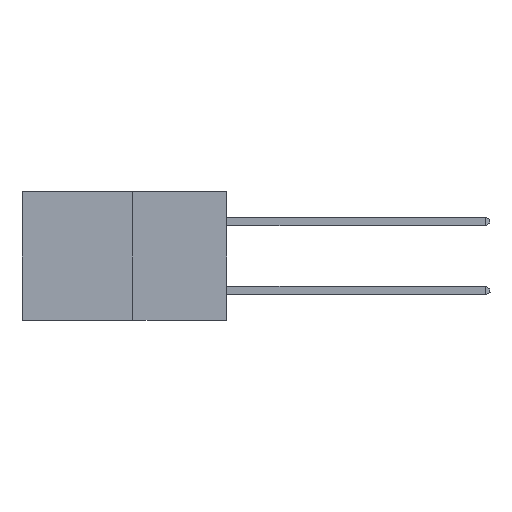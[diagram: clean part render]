
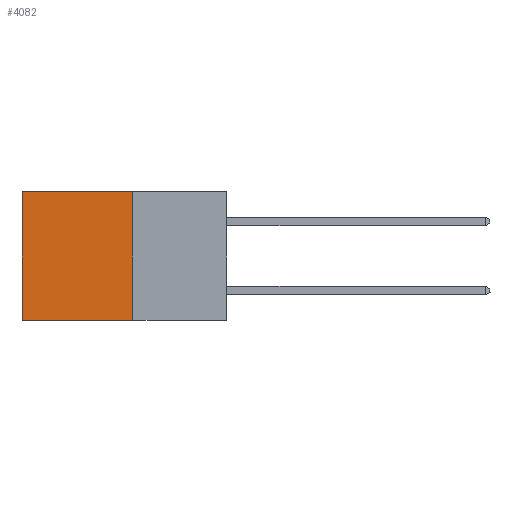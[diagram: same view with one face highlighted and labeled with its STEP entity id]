
A CAD part, left-side view. The second image highlights one B-rep face of the part: STEP entity #4082.
In plain terms, the highlighted planar face has unit normal (-1, 0, 0).
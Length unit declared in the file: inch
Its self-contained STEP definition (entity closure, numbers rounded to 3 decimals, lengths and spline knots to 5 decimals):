
#1865 = LINE ( 'NONE', #2295, #23714 ) ;
#2295 = CARTESIAN_POINT ( 'NONE',  ( 0.277, 0.27, -0.37 ) ) ;
#4072 = CARTESIAN_POINT ( 'NONE',  ( 0.277, 0.59, -0.37 ) ) ;
#4082 = ADVANCED_FACE ( 'NONE', ( #4358 ), #12437, .F. ) ;
#4358 = FACE_OUTER_BOUND ( 'NONE', #25690, .T. ) ;
#4457 = EDGE_CURVE ( 'NONE', #16605, #13602, #10666, .T. ) ;
#4760 = ORIENTED_EDGE ( 'NONE', *, *, #11035, .F. ) ;
#4794 = CARTESIAN_POINT ( 'NONE',  ( 0.277, 0.59, 0. ) ) ;
#5873 = DIRECTION ( 'NONE',  ( 0., 1., 0. ) ) ;
#6000 = CARTESIAN_POINT ( 'NONE',  ( 0.277, 0.27, 0. ) ) ;
#8192 = LINE ( 'NONE', #19286, #25667 ) ;
#9431 = DIRECTION ( 'NONE',  ( 0., 1., 0. ) ) ;
#10104 = AXIS2_PLACEMENT_3D ( 'NONE', #12379, #12317, #12293 ) ;
#10666 = LINE ( 'NONE', #6000, #15632 ) ;
#10964 = LINE ( 'NONE', #24340, #11753 ) ;
#11035 = EDGE_CURVE ( 'NONE', #25923, #20314, #10964, .T. ) ;
#11753 = VECTOR ( 'NONE', #9431, 39.37008 ) ;
#12293 = DIRECTION ( 'NONE',  ( 0., 0., -1. ) ) ;
#12317 = DIRECTION ( 'NONE',  ( 1., 0., 0. ) ) ;
#12379 = CARTESIAN_POINT ( 'NONE',  ( 0.277, 0.27, -0.37 ) ) ;
#12437 = PLANE ( 'NONE',  #10104 ) ;
#13024 = DIRECTION ( 'NONE',  ( 0., 0., -1. ) ) ;
#13602 = VERTEX_POINT ( 'NONE', #4794 ) ;
#15466 = EDGE_CURVE ( 'NONE', #16605, #25923, #1865, .T. ) ;
#15632 = VECTOR ( 'NONE', #5873, 39.37008 ) ;
#15889 = EDGE_CURVE ( 'NONE', #13602, #20314, #8192, .T. ) ;
#16514 = ORIENTED_EDGE ( 'NONE', *, *, #15466, .F. ) ;
#16605 = VERTEX_POINT ( 'NONE', #17299 ) ;
#17299 = CARTESIAN_POINT ( 'NONE',  ( 0.277, 0.27, 0. ) ) ;
#19286 = CARTESIAN_POINT ( 'NONE',  ( 0.277, 0.59, -0.37 ) ) ;
#20314 = VERTEX_POINT ( 'NONE', #4072 ) ;
#20884 = ORIENTED_EDGE ( 'NONE', *, *, #4457, .T. ) ;
#22381 = ORIENTED_EDGE ( 'NONE', *, *, #15889, .T. ) ;
#23476 = DIRECTION ( 'NONE',  ( 0., 0., -1. ) ) ;
#23714 = VECTOR ( 'NONE', #23476, 39.37008 ) ;
#24340 = CARTESIAN_POINT ( 'NONE',  ( 0.277, 0.27, -0.37 ) ) ;
#24460 = CARTESIAN_POINT ( 'NONE',  ( 0.277, 0.27, -0.37 ) ) ;
#25667 = VECTOR ( 'NONE', #13024, 39.37008 ) ;
#25690 = EDGE_LOOP ( 'NONE', ( #22381, #4760, #16514, #20884 ) ) ;
#25923 = VERTEX_POINT ( 'NONE', #24460 ) ;
